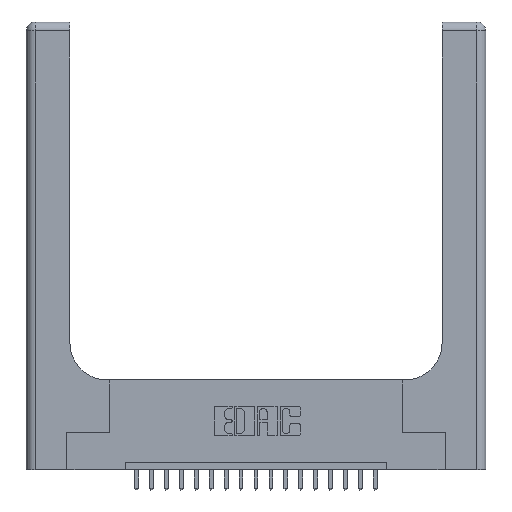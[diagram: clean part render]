
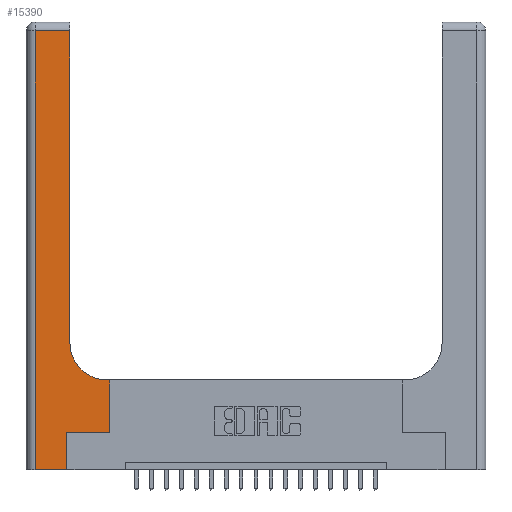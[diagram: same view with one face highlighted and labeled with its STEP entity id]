
A CAD part, top view. The second image highlights one B-rep face of the part: STEP entity #15390.
In plain terms, the highlighted planar face has unit normal (0, 0, 1).
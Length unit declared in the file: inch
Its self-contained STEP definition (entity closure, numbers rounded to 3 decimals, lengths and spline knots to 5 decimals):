
#325 = VECTOR ( 'NONE', #10900, 39.37008 ) ;
#974 = CARTESIAN_POINT ( 'NONE',  ( 0.5585, 0.25, 0.37 ) ) ;
#1458 = CARTESIAN_POINT ( 'NONE',  ( 0.269, 0.25, 0.37 ) ) ;
#1514 = CARTESIAN_POINT ( 'NONE',  ( 0.5585, 0.6, 0.37 ) ) ;
#1701 = VECTOR ( 'NONE', #9358, 39.37008 ) ;
#1709 = ORIENTED_EDGE ( 'NONE', *, *, #8828, .T. ) ;
#1758 = LINE ( 'NONE', #3650, #13109 ) ;
#2074 = CARTESIAN_POINT ( 'NONE',  ( 0.2915, 3., 0.37 ) ) ;
#2282 = DIRECTION ( 'NONE',  ( 0., 0., -1. ) ) ;
#2463 = CARTESIAN_POINT ( 'NONE',  ( 0.269, 0., 0.37 ) ) ;
#2523 = ORIENTED_EDGE ( 'NONE', *, *, #8795, .T. ) ;
#2851 = CARTESIAN_POINT ( 'NONE',  ( 0.06, 3., 0.37 ) ) ;
#3316 = VERTEX_POINT ( 'NONE', #11726 ) ;
#3650 = CARTESIAN_POINT ( 'NONE',  ( 0., 2.94, 0.37 ) ) ;
#3668 = VECTOR ( 'NONE', #9902, 39.37008 ) ;
#3898 = CARTESIAN_POINT ( 'NONE',  ( 0., 3., 0.37 ) ) ;
#3952 = CIRCLE ( 'NONE', #19298, 0.25 ) ;
#4046 = DIRECTION ( 'NONE',  ( -1., 0., 0. ) ) ;
#4285 = EDGE_CURVE ( 'NONE', #3316, #6834, #1758, .T. ) ;
#4619 = VECTOR ( 'NONE', #8818, 39.37008 ) ;
#4755 = DIRECTION ( 'NONE',  ( 1., 0., 0. ) ) ;
#4841 = ORIENTED_EDGE ( 'NONE', *, *, #17678, .T. ) ;
#5628 = EDGE_CURVE ( 'NONE', #6240, #3316, #18541, .T. ) ;
#6240 = VERTEX_POINT ( 'NONE', #13832 ) ;
#6322 = CARTESIAN_POINT ( 'NONE',  ( 0., 0., 0.37 ) ) ;
#6413 = ORIENTED_EDGE ( 'NONE', *, *, #18499, .T. ) ;
#6834 = VERTEX_POINT ( 'NONE', #19334 ) ;
#6996 = ORIENTED_EDGE ( 'NONE', *, *, #4285, .T. ) ;
#8177 = VECTOR ( 'NONE', #12497, 39.37008 ) ;
#8693 = DIRECTION ( 'NONE',  ( -1., 0., 0. ) ) ;
#8710 = VERTEX_POINT ( 'NONE', #20499 ) ;
#8795 = EDGE_CURVE ( 'NONE', #6834, #20166, #16960, .T. ) ;
#8818 = DIRECTION ( 'NONE',  ( 0., 1., 0. ) ) ;
#8828 = EDGE_CURVE ( 'NONE', #8710, #10801, #12282, .T. ) ;
#9061 = AXIS2_PLACEMENT_3D ( 'NONE', #3898, #2282, #4046 ) ;
#9358 = DIRECTION ( 'NONE',  ( 0., -1., 0. ) ) ;
#9404 = DIRECTION ( 'NONE',  ( 1., 0., 0. ) ) ;
#9902 = DIRECTION ( 'NONE',  ( 0., 1., 0. ) ) ;
#9924 = VERTEX_POINT ( 'NONE', #2463 ) ;
#10141 = VECTOR ( 'NONE', #4755, 39.37008 ) ;
#10170 = EDGE_CURVE ( 'NONE', #13595, #8710, #17382, .T. ) ;
#10324 = CARTESIAN_POINT ( 'NONE',  ( 0.269, 0.25, 0.37 ) ) ;
#10801 = VERTEX_POINT ( 'NONE', #1514 ) ;
#10849 = CARTESIAN_POINT ( 'NONE',  ( 0.5415, 0.6, 0.37 ) ) ;
#10874 = LINE ( 'NONE', #14291, #325 ) ;
#10900 = DIRECTION ( 'NONE',  ( -1., 0., 0. ) ) ;
#11726 = CARTESIAN_POINT ( 'NONE',  ( 0.2915, 2.94, 0.37 ) ) ;
#11774 = ORIENTED_EDGE ( 'NONE', *, *, #5628, .T. ) ;
#11797 = EDGE_CURVE ( 'NONE', #9924, #13595, #18891, .T. ) ;
#12282 = LINE ( 'NONE', #974, #8177 ) ;
#12497 = DIRECTION ( 'NONE',  ( 0., 1., 0. ) ) ;
#12517 = ORIENTED_EDGE ( 'NONE', *, *, #10170, .T. ) ;
#12609 = DIRECTION ( 'NONE',  ( 0., 0., -1. ) ) ;
#13109 = VECTOR ( 'NONE', #8693, 39.37008 ) ;
#13173 = EDGE_LOOP ( 'NONE', ( #11774, #6996, #2523, #17450, #20472, #12517, #1709, #4841, #6413 ) ) ;
#13595 = VERTEX_POINT ( 'NONE', #10324 ) ;
#13832 = CARTESIAN_POINT ( 'NONE',  ( 0.2915, 0.85, 0.37 ) ) ;
#14276 = PLANE ( 'NONE',  #9061 ) ;
#14291 = CARTESIAN_POINT ( 'NONE',  ( 0.2915, 0.6, 0.37 ) ) ;
#15284 = CARTESIAN_POINT ( 'NONE',  ( 0.06, 0., 0.37 ) ) ;
#15390 = ADVANCED_FACE ( 'NONE', ( #15865 ), #14276, .F. ) ;
#15865 = FACE_OUTER_BOUND ( 'NONE', #13173, .T. ) ;
#16960 = LINE ( 'NONE', #2851, #1701 ) ;
#17253 = LINE ( 'NONE', #6322, #21334 ) ;
#17382 = LINE ( 'NONE', #1458, #10141 ) ;
#17450 = ORIENTED_EDGE ( 'NONE', *, *, #18956, .T. ) ;
#17678 = EDGE_CURVE ( 'NONE', #10801, #20194, #10874, .T. ) ;
#18142 = CARTESIAN_POINT ( 'NONE',  ( 0.269, 0., 0.37 ) ) ;
#18499 = EDGE_CURVE ( 'NONE', #20194, #6240, #3952, .T. ) ;
#18541 = LINE ( 'NONE', #2074, #4619 ) ;
#18891 = LINE ( 'NONE', #18142, #3668 ) ;
#18956 = EDGE_CURVE ( 'NONE', #20166, #9924, #17253, .T. ) ;
#19273 = CARTESIAN_POINT ( 'NONE',  ( 0.5415, 0.85, 0.37 ) ) ;
#19298 = AXIS2_PLACEMENT_3D ( 'NONE', #19273, #12609, #9404 ) ;
#19334 = CARTESIAN_POINT ( 'NONE',  ( 0.06, 2.94, 0.37 ) ) ;
#19395 = DIRECTION ( 'NONE',  ( 1., 0., 0. ) ) ;
#20166 = VERTEX_POINT ( 'NONE', #15284 ) ;
#20194 = VERTEX_POINT ( 'NONE', #10849 ) ;
#20472 = ORIENTED_EDGE ( 'NONE', *, *, #11797, .T. ) ;
#20499 = CARTESIAN_POINT ( 'NONE',  ( 0.5585, 0.25, 0.37 ) ) ;
#21334 = VECTOR ( 'NONE', #19395, 39.37008 ) ;
